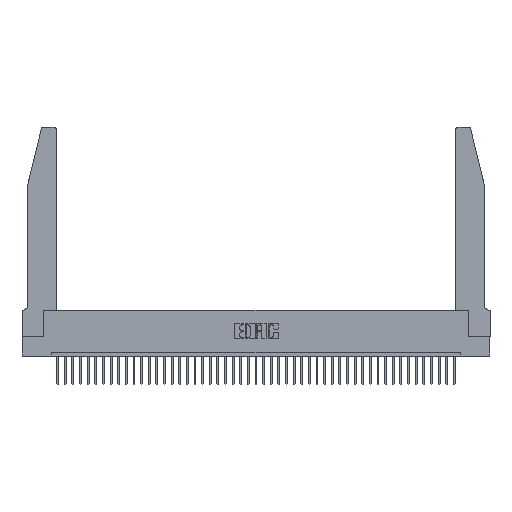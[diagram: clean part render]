
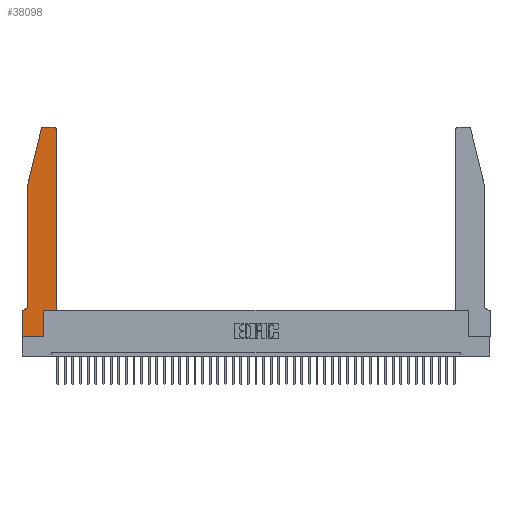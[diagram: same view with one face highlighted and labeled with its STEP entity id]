
A CAD part, top view. The second image highlights one B-rep face of the part: STEP entity #38098.
In plain terms, the highlighted planar face has unit normal (0, 0, 1).
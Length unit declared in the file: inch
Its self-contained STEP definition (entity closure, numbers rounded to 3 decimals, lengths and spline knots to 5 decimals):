
#28 = CARTESIAN_POINT ( 'NONE',  ( 0.0755, 0.42, 0.37 ) ) ;
#704 = VERTEX_POINT ( 'NONE', #41373 ) ;
#1808 = DIRECTION ( 'NONE',  ( 0., 0., 1. ) ) ;
#2027 = CARTESIAN_POINT ( 'NONE',  ( 0.0055, 0.42, 0.37 ) ) ;
#2593 = ORIENTED_EDGE ( 'NONE', *, *, #23510, .T. ) ;
#2985 = DIRECTION ( 'NONE',  ( 1., 0., 0. ) ) ;
#4016 = LINE ( 'NONE', #42615, #8231 ) ;
#5925 = LINE ( 'NONE', #28429, #35126 ) ;
#6056 = DIRECTION ( 'NONE',  ( 0., -1., 0. ) ) ;
#6141 = VECTOR ( 'NONE', #35596, 39.37008 ) ;
#6235 = EDGE_CURVE ( 'NONE', #38960, #9185, #35456, .T. ) ;
#6513 = EDGE_CURVE ( 'NONE', #15683, #35252, #30238, .T. ) ;
#6730 = CIRCLE ( 'NONE', #35208, 0.03 ) ;
#6770 = VERTEX_POINT ( 'NONE', #32027 ) ;
#7272 = VECTOR ( 'NONE', #13552, 39.37008 ) ;
#7739 = ORIENTED_EDGE ( 'NONE', *, *, #16561, .T. ) ;
#8231 = VECTOR ( 'NONE', #6056, 39.37008 ) ;
#8402 = CARTESIAN_POINT ( 'NONE',  ( 0.0755, 0.35, 0.37 ) ) ;
#9120 = ORIENTED_EDGE ( 'NONE', *, *, #40241, .T. ) ;
#9185 = VERTEX_POINT ( 'NONE', #9936 ) ;
#9936 = CARTESIAN_POINT ( 'NONE',  ( 0.4505, 2.72, 0.37 ) ) ;
#10062 = ORIENTED_EDGE ( 'NONE', *, *, #6235, .T. ) ;
#10487 = DIRECTION ( 'NONE',  ( 1., 0., 0. ) ) ;
#12123 = EDGE_CURVE ( 'NONE', #31785, #704, #15665, .T. ) ;
#12202 = AXIS2_PLACEMENT_3D ( 'NONE', #29233, #26176, #2985 ) ;
#12292 = CARTESIAN_POINT ( 'NONE',  ( 0., 0., 0.37 ) ) ;
#13552 = DIRECTION ( 'NONE',  ( 0., 1., 0. ) ) ;
#13756 = VECTOR ( 'NONE', #24869, 39.37008 ) ;
#14015 = VECTOR ( 'NONE', #10487, 39.37008 ) ;
#14086 = EDGE_CURVE ( 'NONE', #9185, #31785, #23869, .T. ) ;
#14195 = CARTESIAN_POINT ( 'NONE',  ( 0.25487, 2.72718, 0.37 ) ) ;
#14691 = DIRECTION ( 'NONE',  ( 1., 0., 0. ) ) ;
#14937 = ORIENTED_EDGE ( 'NONE', *, *, #6513, .T. ) ;
#15169 = CARTESIAN_POINT ( 'NONE',  ( 0., 0.35, 0.37 ) ) ;
#15665 = LINE ( 'NONE', #32491, #27123 ) ;
#15683 = VERTEX_POINT ( 'NONE', #39106 ) ;
#15761 = DIRECTION ( 'NONE',  ( 0., 1., 0. ) ) ;
#16561 = EDGE_CURVE ( 'NONE', #6770, #26983, #31964, .T. ) ;
#17050 = CARTESIAN_POINT ( 'NONE',  ( 0.2865, 0.35, 0.37 ) ) ;
#17489 = CARTESIAN_POINT ( 'NONE',  ( 0.4505, 0.35, 0.37 ) ) ;
#17602 = ORIENTED_EDGE ( 'NONE', *, *, #36791, .T. ) ;
#18467 = CIRCLE ( 'NONE', #30312, 0.07 ) ;
#19303 = ORIENTED_EDGE ( 'NONE', *, *, #19974, .T. ) ;
#19679 = DIRECTION ( 'NONE',  ( -1., 0., 0. ) ) ;
#19847 = VECTOR ( 'NONE', #15761, 39.37008 ) ;
#19974 = EDGE_CURVE ( 'NONE', #704, #30262, #6730, .T. ) ;
#20664 = ORIENTED_EDGE ( 'NONE', *, *, #12123, .T. ) ;
#22173 = DIRECTION ( 'NONE',  ( -1., 0., 0. ) ) ;
#22441 = ORIENTED_EDGE ( 'NONE', *, *, #36441, .T. ) ;
#23510 = EDGE_CURVE ( 'NONE', #28150, #6770, #18467, .T. ) ;
#23576 = EDGE_CURVE ( 'NONE', #30262, #25098, #5925, .T. ) ;
#23869 = CIRCLE ( 'NONE', #12202, 0.03 ) ;
#24040 = ORIENTED_EDGE ( 'NONE', *, *, #23576, .T. ) ;
#24741 = DIRECTION ( 'NONE',  ( 1., 0., 0. ) ) ;
#24778 = FACE_OUTER_BOUND ( 'NONE', #38857, .T. ) ;
#24869 = DIRECTION ( 'NONE',  ( -1., 0., 0. ) ) ;
#24978 = CARTESIAN_POINT ( 'NONE',  ( 0.2865, 0.35, 0.37 ) ) ;
#25046 = PLANE ( 'NONE',  #26508 ) ;
#25098 = VERTEX_POINT ( 'NONE', #34795 ) ;
#25984 = LINE ( 'NONE', #12292, #6141 ) ;
#26176 = DIRECTION ( 'NONE',  ( 0., 0., 1. ) ) ;
#26508 = AXIS2_PLACEMENT_3D ( 'NONE', #15169, #42078, #41647 ) ;
#26983 = VERTEX_POINT ( 'NONE', #31708 ) ;
#27123 = VECTOR ( 'NONE', #19679, 39.37008 ) ;
#27482 = VERTEX_POINT ( 'NONE', #37463 ) ;
#28150 = VERTEX_POINT ( 'NONE', #28 ) ;
#28213 = ORIENTED_EDGE ( 'NONE', *, *, #14086, .T. ) ;
#28235 = CARTESIAN_POINT ( 'NONE',  ( 0., 0., 0.37 ) ) ;
#28429 = CARTESIAN_POINT ( 'NONE',  ( 0.0755, 2., 0.37 ) ) ;
#29233 = CARTESIAN_POINT ( 'NONE',  ( 0.4205, 2.72, 0.37 ) ) ;
#29710 = CARTESIAN_POINT ( 'NONE',  ( 0.4505, 0.35, 0.37 ) ) ;
#30238 = LINE ( 'NONE', #17050, #7272 ) ;
#30262 = VERTEX_POINT ( 'NONE', #14195 ) ;
#30312 = AXIS2_PLACEMENT_3D ( 'NONE', #2027, #31939, #22173 ) ;
#30660 = CARTESIAN_POINT ( 'NONE',  ( 0.4205, 2.75, 0.37 ) ) ;
#31570 = ORIENTED_EDGE ( 'NONE', *, *, #41441, .T. ) ;
#31708 = CARTESIAN_POINT ( 'NONE',  ( 0., 0.35, 0.37 ) ) ;
#31785 = VERTEX_POINT ( 'NONE', #30660 ) ;
#31939 = DIRECTION ( 'NONE',  ( 0., 0., -1. ) ) ;
#31964 = LINE ( 'NONE', #8402, #13756 ) ;
#32027 = CARTESIAN_POINT ( 'NONE',  ( 0.0055, 0.35, 0.37 ) ) ;
#32491 = CARTESIAN_POINT ( 'NONE',  ( 0.2605, 2.75, 0.37 ) ) ;
#32790 = LINE ( 'NONE', #17489, #14015 ) ;
#33310 = CARTESIAN_POINT ( 'NONE',  ( 0.4505, 0.35, 0.37 ) ) ;
#34795 = CARTESIAN_POINT ( 'NONE',  ( 0.0755, 2., 0.37 ) ) ;
#35126 = VECTOR ( 'NONE', #41975, 39.37008 ) ;
#35208 = AXIS2_PLACEMENT_3D ( 'NONE', #38565, #1808, #14691 ) ;
#35252 = VERTEX_POINT ( 'NONE', #24978 ) ;
#35456 = LINE ( 'NONE', #29710, #19847 ) ;
#35596 = DIRECTION ( 'NONE',  ( 0., -1., 0. ) ) ;
#36441 = EDGE_CURVE ( 'NONE', #35252, #38960, #32790, .T. ) ;
#36791 = EDGE_CURVE ( 'NONE', #25098, #28150, #4016, .T. ) ;
#37463 = CARTESIAN_POINT ( 'NONE',  ( 0., 0., 0.37 ) ) ;
#38098 = ADVANCED_FACE ( 'NONE', ( #24778 ), #25046, .T. ) ;
#38565 = CARTESIAN_POINT ( 'NONE',  ( 0.284, 2.72, 0.37 ) ) ;
#38857 = EDGE_LOOP ( 'NONE', ( #20664, #19303, #24040, #17602, #2593, #7739, #31570, #9120, #14937, #22441, #10062, #28213 ) ) ;
#38960 = VERTEX_POINT ( 'NONE', #33310 ) ;
#39063 = LINE ( 'NONE', #28235, #42651 ) ;
#39106 = CARTESIAN_POINT ( 'NONE',  ( 0.2865, 0., 0.37 ) ) ;
#40241 = EDGE_CURVE ( 'NONE', #27482, #15683, #39063, .T. ) ;
#41373 = CARTESIAN_POINT ( 'NONE',  ( 0.284, 2.75, 0.37 ) ) ;
#41441 = EDGE_CURVE ( 'NONE', #26983, #27482, #25984, .T. ) ;
#41647 = DIRECTION ( 'NONE',  ( 1., 0., 0. ) ) ;
#41975 = DIRECTION ( 'NONE',  ( -0.239, -0.971, 0. ) ) ;
#42078 = DIRECTION ( 'NONE',  ( 0., 0., 1. ) ) ;
#42615 = CARTESIAN_POINT ( 'NONE',  ( 0.0755, 2., 0.37 ) ) ;
#42651 = VECTOR ( 'NONE', #24741, 39.37008 ) ;
